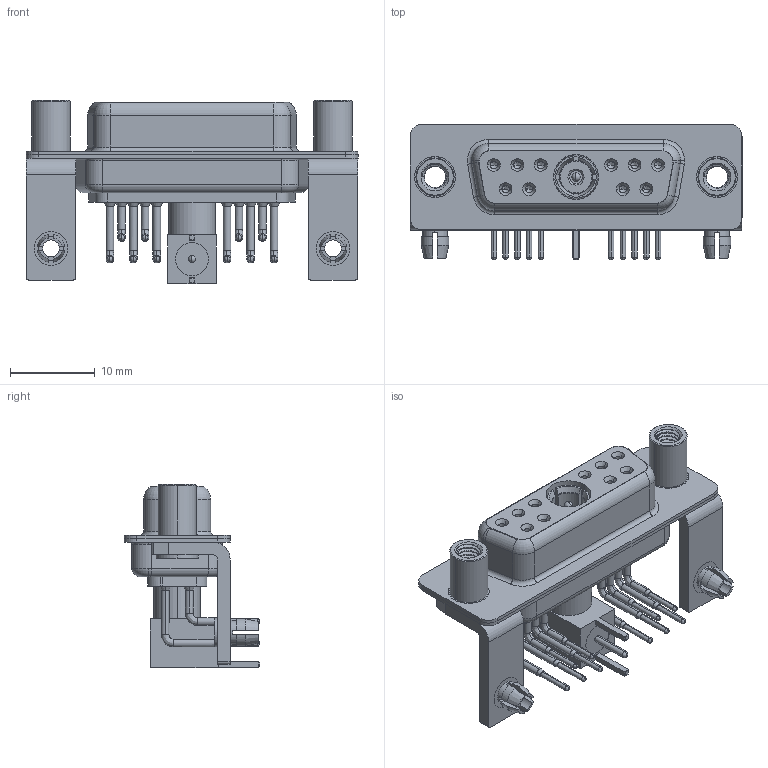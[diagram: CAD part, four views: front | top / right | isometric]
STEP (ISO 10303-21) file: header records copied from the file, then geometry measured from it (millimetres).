
FILE_DESCRIPTION (( 'STEP AP203' ), '1' );
FILE_NAME ('630-11W1640-7ND.STEP', '2022-05-31T14:43:00', ( '' ), ( '' ), 'SwSTEP 2.0', 'SolidWorks 2020', '' );
FILE_SCHEMA (( 'CONFIG_CONTROL_DESIGN' ));
Length unit declared in the file: millimetre
Products named in the file (16): Insulator RA Pin; 630Combo Housing_11W1; Pin_RA; 630-11W1640-7ND; 630Combo Shell Rear_15 Contacts; Co-Ax Plug Assy_RA; 630Combo Shell Front_15 Contacts; Co-Ax Plug_RA PC Tail; 630Combo Threaded Standoff_D; Insulator Pin_Straight PC Tail; Locking Collar; 630Combo Stabilizer Bracket; 630Combo Contact Row 2; RA Back Shell; 630Combo Board Lock; 630Combo Contact Row 1
Assembly tree (26 placements, depth 3):
  630-11W1640-7ND
    630Combo Housing_11W1
    630Combo Shell Front_15 Contacts
    630Combo Shell Rear_15 Contacts
    630Combo Stabilizer Bracket  x2
    630Combo Board Lock  x2
    630Combo Threaded Standoff_D  x2
    Co-Ax Plug Assy_RA
      Co-Ax Plug_RA PC Tail
      Insulator Pin_Straight PC Tail
      Pin_RA
      Locking Collar
      RA Back Shell
      Insulator RA Pin
    630Combo Contact Row 1  x6
    630Combo Contact Row 2  x4
Bounding box: 39.2 x 16 x 21.61 mm (x, y, z)
Volume: 3231.8 mm3; surface area: 8028.4 mm2
Topology: 25 solids, 25 shells, 1167 faces, 2950 edges, 1866 vertices
Faces by surface type: cylinder 536, plane 354, cone 163, torus 63, bspline 47, sphere 4
Entity records: 25823 total; most frequent: CARTESIAN_POINT 6565, DIRECTION 3864, ORIENTED_EDGE 3472, EDGE_CURVE 1736, AXIS2_PLACEMENT_3D 1561, VERTEX_POINT 1107, EDGE_LOOP 831, CIRCLE 824
